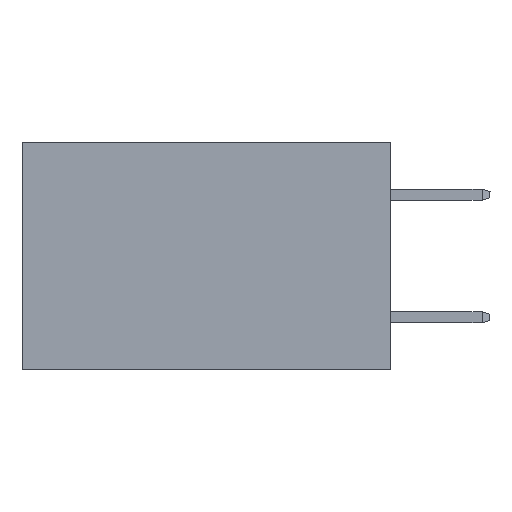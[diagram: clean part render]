
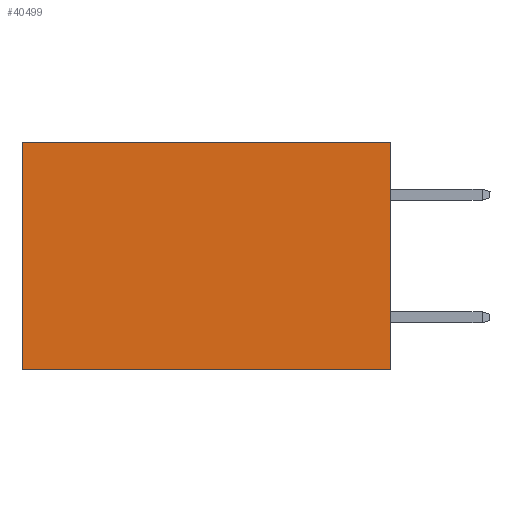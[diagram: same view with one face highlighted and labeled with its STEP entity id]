
A CAD part, left-side view. The second image highlights one B-rep face of the part: STEP entity #40499.
In plain terms, the highlighted planar face has unit normal (-1, 0, 0).
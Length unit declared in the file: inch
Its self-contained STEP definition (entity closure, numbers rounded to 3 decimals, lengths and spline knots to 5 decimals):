
#2305 = CARTESIAN_POINT ( 'NONE',  ( 0.2875, 0., 0. ) ) ;
#2692 = VECTOR ( 'NONE', #40322, 39.37008 ) ;
#4500 = EDGE_CURVE ( 'NONE', #40586, #28953, #35214, .T. ) ;
#5151 = PLANE ( 'NONE',  #31787 ) ;
#7733 = CARTESIAN_POINT ( 'NONE',  ( 0.2875, 0., -0.37 ) ) ;
#8551 = ORIENTED_EDGE ( 'NONE', *, *, #17171, .T. ) ;
#9022 = CARTESIAN_POINT ( 'NONE',  ( 0.2875, 0., -0.37 ) ) ;
#9964 = ORIENTED_EDGE ( 'NONE', *, *, #13649, .F. ) ;
#11065 = CARTESIAN_POINT ( 'NONE',  ( 0.2875, 0., 0. ) ) ;
#11905 = VECTOR ( 'NONE', #32807, 39.37008 ) ;
#12041 = CARTESIAN_POINT ( 'NONE',  ( 0.2875, 0.6, -0.37 ) ) ;
#13621 = EDGE_LOOP ( 'NONE', ( #28049, #9964, #36899, #8551 ) ) ;
#13649 = EDGE_CURVE ( 'NONE', #21060, #28953, #16593, .T. ) ;
#14608 = CARTESIAN_POINT ( 'NONE',  ( 0.2875, 0., 0. ) ) ;
#16508 = EDGE_CURVE ( 'NONE', #20318, #21060, #29290, .T. ) ;
#16593 = LINE ( 'NONE', #7733, #2692 ) ;
#17171 = EDGE_CURVE ( 'NONE', #20318, #40586, #33771, .T. ) ;
#18497 = CARTESIAN_POINT ( 'NONE',  ( 0.2875, 0., 0. ) ) ;
#19839 = VECTOR ( 'NONE', #24890, 39.37008 ) ;
#20318 = VERTEX_POINT ( 'NONE', #2305 ) ;
#21060 = VERTEX_POINT ( 'NONE', #9022 ) ;
#23851 = DIRECTION ( 'NONE',  ( 0., 1., 0. ) ) ;
#24727 = CARTESIAN_POINT ( 'NONE',  ( 0.2875, 0.6, 0. ) ) ;
#24890 = DIRECTION ( 'NONE',  ( 0., 0., -1. ) ) ;
#27416 = DIRECTION ( 'NONE',  ( 1., 0., 0. ) ) ;
#28049 = ORIENTED_EDGE ( 'NONE', *, *, #4500, .T. ) ;
#28953 = VERTEX_POINT ( 'NONE', #12041 ) ;
#29290 = LINE ( 'NONE', #18497, #19839 ) ;
#31787 = AXIS2_PLACEMENT_3D ( 'NONE', #14608, #27416, #33946 ) ;
#32807 = DIRECTION ( 'NONE',  ( 0., 0., -1. ) ) ;
#33771 = LINE ( 'NONE', #11065, #38207 ) ;
#33946 = DIRECTION ( 'NONE',  ( 0., 0., -1. ) ) ;
#35214 = LINE ( 'NONE', #38964, #11905 ) ;
#36899 = ORIENTED_EDGE ( 'NONE', *, *, #16508, .F. ) ;
#38207 = VECTOR ( 'NONE', #23851, 39.37008 ) ;
#38499 = FACE_OUTER_BOUND ( 'NONE', #13621, .T. ) ;
#38964 = CARTESIAN_POINT ( 'NONE',  ( 0.2875, 0.6, 0. ) ) ;
#40322 = DIRECTION ( 'NONE',  ( 0., 1., 0. ) ) ;
#40499 = ADVANCED_FACE ( 'NONE', ( #38499 ), #5151, .F. ) ;
#40586 = VERTEX_POINT ( 'NONE', #24727 ) ;
